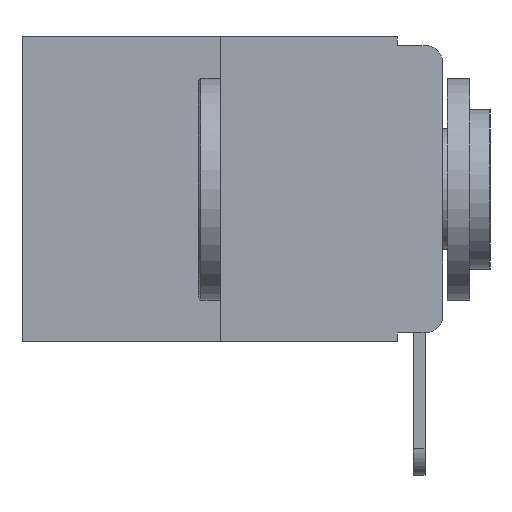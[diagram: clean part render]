
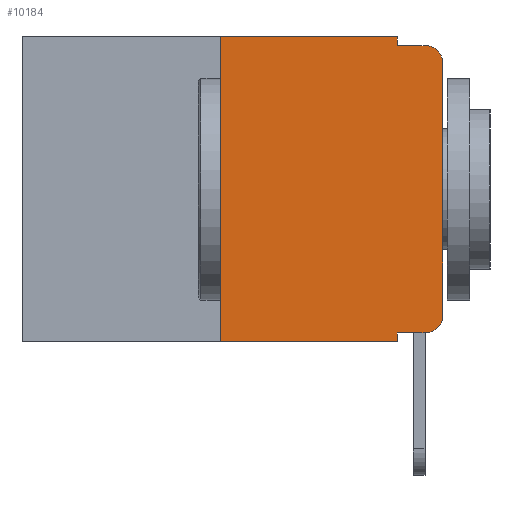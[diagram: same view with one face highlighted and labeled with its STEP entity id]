
A CAD part, left-side view. The second image highlights one B-rep face of the part: STEP entity #10184.
In plain terms, the highlighted planar face has unit normal (-1, 0, 0).
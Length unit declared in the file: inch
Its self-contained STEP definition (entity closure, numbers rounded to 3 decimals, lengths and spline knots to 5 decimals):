
#72 = CARTESIAN_POINT ( 'NONE',  ( 0., 0.473, 0. ) ) ;
#83 = ORIENTED_EDGE ( 'NONE', *, *, #4058, .T. ) ;
#139 = CARTESIAN_POINT ( 'NONE',  ( 0., 0.02, -0.333 ) ) ;
#731 = LINE ( 'NONE', #8881, #6337 ) ;
#786 = ORIENTED_EDGE ( 'NONE', *, *, #3296, .T. ) ;
#1239 = ORIENTED_EDGE ( 'NONE', *, *, #7567, .F. ) ;
#1262 = VECTOR ( 'NONE', #4336, 39.37008 ) ;
#1779 = EDGE_LOOP ( 'NONE', ( #3087, #6249, #6564, #12761, #3242, #1239, #3208, #4207, #83, #786 ) ) ;
#1855 = VERTEX_POINT ( 'NONE', #5929 ) ;
#1859 = FACE_OUTER_BOUND ( 'NONE', #1779, .T. ) ;
#1872 = VECTOR ( 'NONE', #5991, 39.37008 ) ;
#2447 = CARTESIAN_POINT ( 'NONE',  ( 0., 0.051, -0.343 ) ) ;
#2544 = DIRECTION ( 'NONE',  ( 0., 0., -1. ) ) ;
#2624 = VERTEX_POINT ( 'NONE', #2447 ) ;
#2650 = DIRECTION ( 'NONE',  ( 0., -1., 0. ) ) ;
#2952 = LINE ( 'NONE', #3852, #1872 ) ;
#3087 = ORIENTED_EDGE ( 'NONE', *, *, #12809, .T. ) ;
#3208 = ORIENTED_EDGE ( 'NONE', *, *, #7934, .T. ) ;
#3242 = ORIENTED_EDGE ( 'NONE', *, *, #5955, .F. ) ;
#3296 = EDGE_CURVE ( 'NONE', #9513, #3710, #10796, .T. ) ;
#3394 = CARTESIAN_POINT ( 'NONE',  ( 0., 0.051, -0.333 ) ) ;
#3657 = DIRECTION ( 'NONE',  ( 0., -1., 0. ) ) ;
#3710 = VERTEX_POINT ( 'NONE', #8124 ) ;
#3852 = CARTESIAN_POINT ( 'NONE',  ( 0., 0.473, -0.343 ) ) ;
#3919 = DIRECTION ( 'NONE',  ( 0., 0., -1. ) ) ;
#4058 = EDGE_CURVE ( 'NONE', #5813, #9513, #4583, .T. ) ;
#4156 = CIRCLE ( 'NONE', #6763, 0.02 ) ;
#4207 = ORIENTED_EDGE ( 'NONE', *, *, #4755, .F. ) ;
#4336 = DIRECTION ( 'NONE',  ( 0., -1., 0. ) ) ;
#4368 = VERTEX_POINT ( 'NONE', #6955 ) ;
#4494 = VECTOR ( 'NONE', #3919, 39.37008 ) ;
#4583 = LINE ( 'NONE', #3394, #10029 ) ;
#4755 = EDGE_CURVE ( 'NONE', #5813, #2624, #8773, .T. ) ;
#4786 = DIRECTION ( 'NONE',  ( -1., 0., 0. ) ) ;
#4889 = VERTEX_POINT ( 'NONE', #10561 ) ;
#4953 = CARTESIAN_POINT ( 'NONE',  ( 0., 0.02, -0.313 ) ) ;
#5116 = DIRECTION ( 'NONE',  ( 0., 0., -1. ) ) ;
#5185 = CARTESIAN_POINT ( 'NONE',  ( 0., 0.25, 0. ) ) ;
#5218 = DIRECTION ( 'NONE',  ( -1., 0., 0. ) ) ;
#5813 = VERTEX_POINT ( 'NONE', #7693 ) ;
#5929 = CARTESIAN_POINT ( 'NONE',  ( 0., 0.02, -0.01 ) ) ;
#5955 = EDGE_CURVE ( 'NONE', #4368, #4889, #731, .T. ) ;
#5991 = DIRECTION ( 'NONE',  ( 0., -1., 0. ) ) ;
#6249 = ORIENTED_EDGE ( 'NONE', *, *, #10236, .T. ) ;
#6250 = CARTESIAN_POINT ( 'NONE',  ( 0., 0.25, -0.343 ) ) ;
#6315 = LINE ( 'NONE', #5185, #9369 ) ;
#6337 = VECTOR ( 'NONE', #3657, 39.37008 ) ;
#6564 = ORIENTED_EDGE ( 'NONE', *, *, #8265, .F. ) ;
#6712 = LINE ( 'NONE', #7622, #11701 ) ;
#6763 = AXIS2_PLACEMENT_3D ( 'NONE', #10868, #4786, #11851 ) ;
#6794 = VERTEX_POINT ( 'NONE', #10907 ) ;
#6955 = CARTESIAN_POINT ( 'NONE',  ( 0., 0.25, 0. ) ) ;
#7066 = VERTEX_POINT ( 'NONE', #6250 ) ;
#7480 = AXIS2_PLACEMENT_3D ( 'NONE', #72, #8876, #2544 ) ;
#7567 = EDGE_CURVE ( 'NONE', #7066, #4368, #6315, .T. ) ;
#7603 = AXIS2_PLACEMENT_3D ( 'NONE', #4953, #5218, #5116 ) ;
#7622 = CARTESIAN_POINT ( 'NONE',  ( 0., 0., 0. ) ) ;
#7693 = CARTESIAN_POINT ( 'NONE',  ( 0., 0.051, -0.333 ) ) ;
#7730 = CARTESIAN_POINT ( 'NONE',  ( 0., 0.051, -0.01 ) ) ;
#7934 = EDGE_CURVE ( 'NONE', #7066, #2624, #2952, .T. ) ;
#8100 = CARTESIAN_POINT ( 'NONE',  ( 0., 0.051, 0. ) ) ;
#8124 = CARTESIAN_POINT ( 'NONE',  ( 0., 0., -0.313 ) ) ;
#8265 = EDGE_CURVE ( 'NONE', #10095, #1855, #9808, .T. ) ;
#8508 = DIRECTION ( 'NONE',  ( 0., 0., -1. ) ) ;
#8642 = DIRECTION ( 'NONE',  ( 0., 0., 1. ) ) ;
#8773 = LINE ( 'NONE', #10487, #11059 ) ;
#8876 = DIRECTION ( 'NONE',  ( 1., 0., 0. ) ) ;
#8881 = CARTESIAN_POINT ( 'NONE',  ( 0., 0.473, 0. ) ) ;
#9369 = VECTOR ( 'NONE', #12189, 39.37008 ) ;
#9484 = CARTESIAN_POINT ( 'NONE',  ( 0., 0.051, -0.01 ) ) ;
#9513 = VERTEX_POINT ( 'NONE', #139 ) ;
#9601 = EDGE_CURVE ( 'NONE', #4889, #10095, #12507, .T. ) ;
#9808 = LINE ( 'NONE', #9484, #1262 ) ;
#10029 = VECTOR ( 'NONE', #2650, 39.37008 ) ;
#10095 = VERTEX_POINT ( 'NONE', #7730 ) ;
#10184 = ADVANCED_FACE ( 'NONE', ( #1859 ), #12721, .F. ) ;
#10236 = EDGE_CURVE ( 'NONE', #6794, #1855, #4156, .T. ) ;
#10487 = CARTESIAN_POINT ( 'NONE',  ( 0., 0.051, 0. ) ) ;
#10561 = CARTESIAN_POINT ( 'NONE',  ( 0., 0.051, 0. ) ) ;
#10796 = CIRCLE ( 'NONE', #7603, 0.02 ) ;
#10868 = CARTESIAN_POINT ( 'NONE',  ( 0., 0.02, -0.03 ) ) ;
#10907 = CARTESIAN_POINT ( 'NONE',  ( 0., 0., -0.03 ) ) ;
#11059 = VECTOR ( 'NONE', #8508, 39.37008 ) ;
#11701 = VECTOR ( 'NONE', #8642, 39.37008 ) ;
#11851 = DIRECTION ( 'NONE',  ( 0., 0., -1. ) ) ;
#12189 = DIRECTION ( 'NONE',  ( 0., 0., 1. ) ) ;
#12507 = LINE ( 'NONE', #8100, #4494 ) ;
#12721 = PLANE ( 'NONE',  #7480 ) ;
#12761 = ORIENTED_EDGE ( 'NONE', *, *, #9601, .F. ) ;
#12809 = EDGE_CURVE ( 'NONE', #3710, #6794, #6712, .T. ) ;
